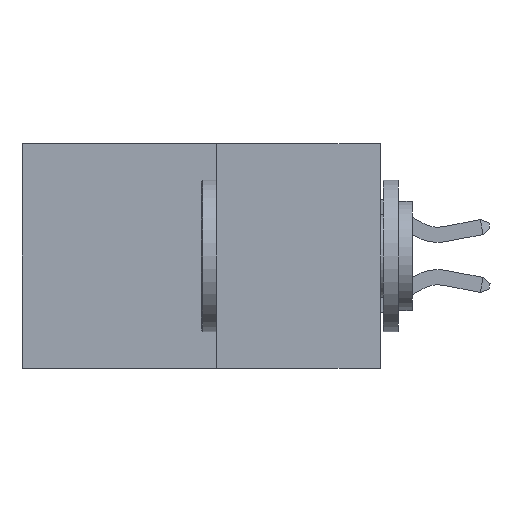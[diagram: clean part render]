
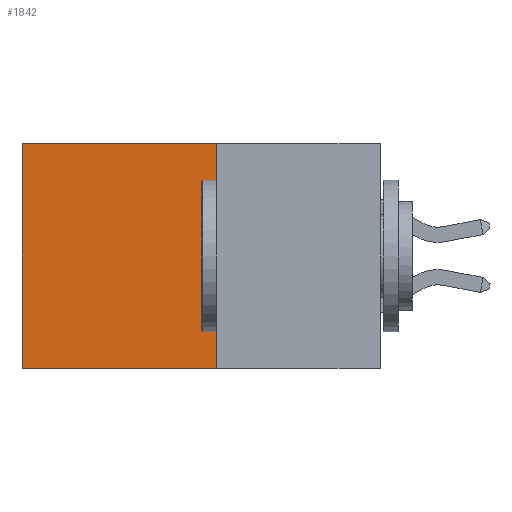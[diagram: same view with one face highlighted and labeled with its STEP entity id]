
A CAD part, left-side view. The second image highlights one B-rep face of the part: STEP entity #1842.
In plain terms, the highlighted planar face has unit normal (-1, 0, 0).
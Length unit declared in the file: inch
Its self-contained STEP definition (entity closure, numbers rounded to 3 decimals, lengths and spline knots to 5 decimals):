
#211 = LINE ( 'NONE', #636, #4054 ) ;
#636 = CARTESIAN_POINT ( 'NONE',  ( 0.277, 0.27, -0.37 ) ) ;
#1191 = LINE ( 'NONE', #8555, #3290 ) ;
#1365 = FACE_OUTER_BOUND ( 'NONE', #4786, .T. ) ;
#1400 = DIRECTION ( 'NONE',  ( 0., 1., 0. ) ) ;
#1842 = ADVANCED_FACE ( 'NONE', ( #1365 ), #3032, .F. ) ;
#2142 = ORIENTED_EDGE ( 'NONE', *, *, #3489, .T. ) ;
#2523 = CARTESIAN_POINT ( 'NONE',  ( 0.277, 0.27, -0.37 ) ) ;
#2594 = LINE ( 'NONE', #3287, #6715 ) ;
#3032 = PLANE ( 'NONE',  #4966 ) ;
#3287 = CARTESIAN_POINT ( 'NONE',  ( 0.277, 0.59, -0.37 ) ) ;
#3290 = VECTOR ( 'NONE', #8536, 39.37008 ) ;
#3489 = EDGE_CURVE ( 'NONE', #5159, #6661, #1191, .T. ) ;
#3657 = DIRECTION ( 'NONE',  ( 0., 0., -1. ) ) ;
#3709 = CARTESIAN_POINT ( 'NONE',  ( 0.277, 0.59, 0. ) ) ;
#3936 = ORIENTED_EDGE ( 'NONE', *, *, #7095, .F. ) ;
#4054 = VECTOR ( 'NONE', #1400, 39.37008 ) ;
#4296 = DIRECTION ( 'NONE',  ( 1., 0., 0. ) ) ;
#4401 = CARTESIAN_POINT ( 'NONE',  ( 0.277, 0.27, 0. ) ) ;
#4613 = VERTEX_POINT ( 'NONE', #7570 ) ;
#4657 = CARTESIAN_POINT ( 'NONE',  ( 0.277, 0.27, -0.37 ) ) ;
#4786 = EDGE_LOOP ( 'NONE', ( #5508, #3936, #5723, #2142 ) ) ;
#4966 = AXIS2_PLACEMENT_3D ( 'NONE', #2523, #4296, #8280 ) ;
#5159 = VERTEX_POINT ( 'NONE', #4401 ) ;
#5229 = EDGE_CURVE ( 'NONE', #6661, #7911, #2594, .T. ) ;
#5328 = DIRECTION ( 'NONE',  ( 0., 0., -1. ) ) ;
#5508 = ORIENTED_EDGE ( 'NONE', *, *, #5229, .T. ) ;
#5723 = ORIENTED_EDGE ( 'NONE', *, *, #7232, .F. ) ;
#6661 = VERTEX_POINT ( 'NONE', #3709 ) ;
#6715 = VECTOR ( 'NONE', #3657, 39.37008 ) ;
#7095 = EDGE_CURVE ( 'NONE', #4613, #7911, #211, .T. ) ;
#7232 = EDGE_CURVE ( 'NONE', #5159, #4613, #7458, .T. ) ;
#7458 = LINE ( 'NONE', #4657, #8668 ) ;
#7570 = CARTESIAN_POINT ( 'NONE',  ( 0.277, 0.27, -0.37 ) ) ;
#7712 = CARTESIAN_POINT ( 'NONE',  ( 0.277, 0.59, -0.37 ) ) ;
#7911 = VERTEX_POINT ( 'NONE', #7712 ) ;
#8280 = DIRECTION ( 'NONE',  ( 0., 0., -1. ) ) ;
#8536 = DIRECTION ( 'NONE',  ( 0., 1., 0. ) ) ;
#8555 = CARTESIAN_POINT ( 'NONE',  ( 0.277, 0.27, 0. ) ) ;
#8668 = VECTOR ( 'NONE', #5328, 39.37008 ) ;
